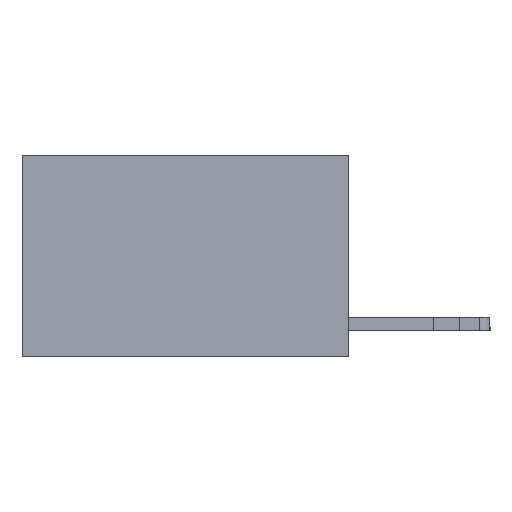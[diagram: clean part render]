
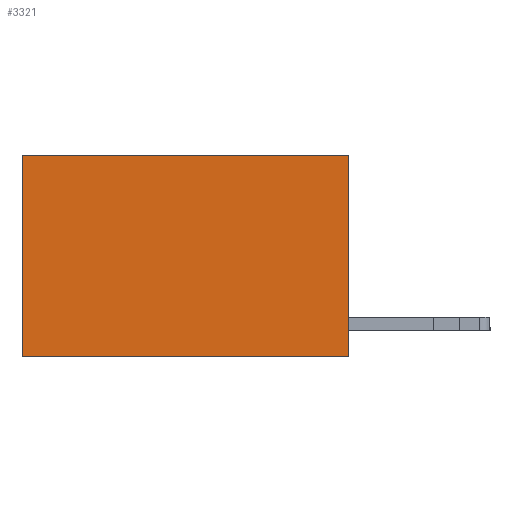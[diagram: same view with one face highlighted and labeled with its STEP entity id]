
A CAD part, left-side view. The second image highlights one B-rep face of the part: STEP entity #3321.
In plain terms, the highlighted planar face has unit normal (-1, 0, 0).
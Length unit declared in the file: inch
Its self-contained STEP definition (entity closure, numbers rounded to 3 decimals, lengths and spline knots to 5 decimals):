
#444 = VERTEX_POINT ( 'NONE', #6679 ) ;
#533 = ORIENTED_EDGE ( 'NONE', *, *, #15044, .F. ) ;
#831 = ORIENTED_EDGE ( 'NONE', *, *, #13201, .T. ) ;
#2197 = CARTESIAN_POINT ( 'NONE',  ( 0.2625, 0., -0.37 ) ) ;
#2600 = VECTOR ( 'NONE', #9046, 39.37008 ) ;
#3321 = ADVANCED_FACE ( 'NONE', ( #6643 ), #17656, .F. ) ;
#3461 = DIRECTION ( 'NONE',  ( 0., 0., -1. ) ) ;
#3613 = VERTEX_POINT ( 'NONE', #2197 ) ;
#4884 = CARTESIAN_POINT ( 'NONE',  ( 0.2625, 0.6, 0. ) ) ;
#4941 = LINE ( 'NONE', #10446, #9917 ) ;
#4963 = CARTESIAN_POINT ( 'NONE',  ( 0.2625, 0., 0. ) ) ;
#5469 = DIRECTION ( 'NONE',  ( 1., 0., 0. ) ) ;
#6267 = EDGE_LOOP ( 'NONE', ( #16430, #533, #16001, #831 ) ) ;
#6525 = EDGE_CURVE ( 'NONE', #15920, #3613, #9868, .T. ) ;
#6559 = VECTOR ( 'NONE', #3461, 39.37008 ) ;
#6643 = FACE_OUTER_BOUND ( 'NONE', #6267, .T. ) ;
#6679 = CARTESIAN_POINT ( 'NONE',  ( 0.2625, 0.6, -0.37 ) ) ;
#7338 = CARTESIAN_POINT ( 'NONE',  ( 0.2625, 0.6, 0. ) ) ;
#8235 = VECTOR ( 'NONE', #17728, 39.37008 ) ;
#9046 = DIRECTION ( 'NONE',  ( 0., 0., -1. ) ) ;
#9438 = LINE ( 'NONE', #9524, #8235 ) ;
#9444 = CARTESIAN_POINT ( 'NONE',  ( 0.2625, 0., 0. ) ) ;
#9524 = CARTESIAN_POINT ( 'NONE',  ( 0.2625, 0., -0.37 ) ) ;
#9868 = LINE ( 'NONE', #10399, #2600 ) ;
#9917 = VECTOR ( 'NONE', #13105, 39.37008 ) ;
#10399 = CARTESIAN_POINT ( 'NONE',  ( 0.2625, 0., 0. ) ) ;
#10446 = CARTESIAN_POINT ( 'NONE',  ( 0.2625, 0., 0. ) ) ;
#10788 = DIRECTION ( 'NONE',  ( 0., 0., -1. ) ) ;
#11235 = AXIS2_PLACEMENT_3D ( 'NONE', #9444, #5469, #10788 ) ;
#13105 = DIRECTION ( 'NONE',  ( 0., 1., 0. ) ) ;
#13201 = EDGE_CURVE ( 'NONE', #15920, #17285, #4941, .T. ) ;
#15044 = EDGE_CURVE ( 'NONE', #3613, #444, #9438, .T. ) ;
#15538 = LINE ( 'NONE', #7338, #6559 ) ;
#15920 = VERTEX_POINT ( 'NONE', #4963 ) ;
#16001 = ORIENTED_EDGE ( 'NONE', *, *, #6525, .F. ) ;
#16430 = ORIENTED_EDGE ( 'NONE', *, *, #16657, .T. ) ;
#16657 = EDGE_CURVE ( 'NONE', #17285, #444, #15538, .T. ) ;
#17285 = VERTEX_POINT ( 'NONE', #4884 ) ;
#17656 = PLANE ( 'NONE',  #11235 ) ;
#17728 = DIRECTION ( 'NONE',  ( 0., 1., 0. ) ) ;
